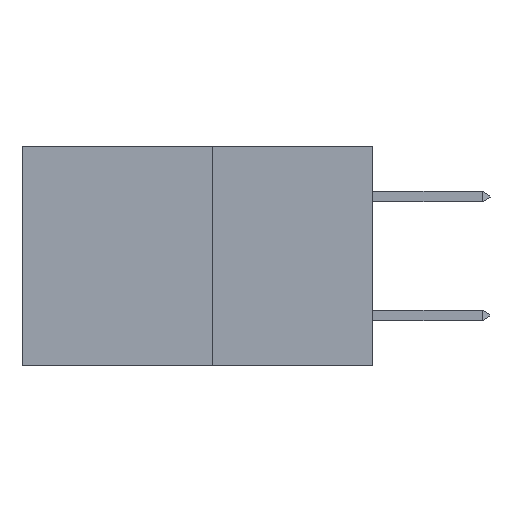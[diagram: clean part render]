
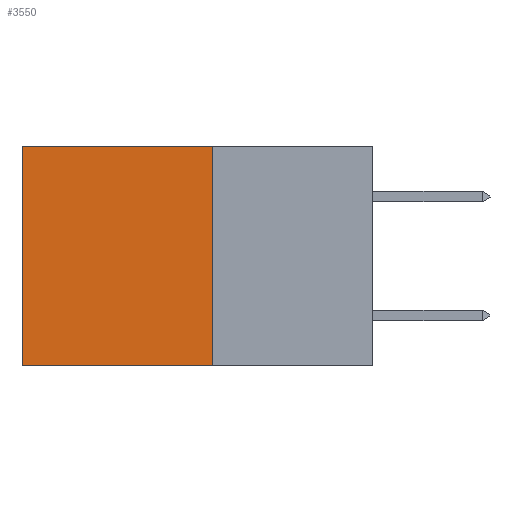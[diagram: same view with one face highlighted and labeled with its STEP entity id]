
A CAD part, left-side view. The second image highlights one B-rep face of the part: STEP entity #3550.
In plain terms, the highlighted planar face has unit normal (-1, 0, 0).
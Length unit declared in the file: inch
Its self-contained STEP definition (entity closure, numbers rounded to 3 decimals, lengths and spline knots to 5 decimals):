
#51 = CARTESIAN_POINT ( 'NONE',  ( 0.277, 0.27, -0.37 ) ) ;
#347 = LINE ( 'NONE', #5364, #7031 ) ;
#578 = EDGE_CURVE ( 'NONE', #8061, #8725, #347, .T. ) ;
#642 = EDGE_CURVE ( 'NONE', #658, #8061, #9654, .T. ) ;
#658 = VERTEX_POINT ( 'NONE', #11621 ) ;
#836 = ORIENTED_EDGE ( 'NONE', *, *, #642, .T. ) ;
#2656 = VECTOR ( 'NONE', #3033, 39.37008 ) ;
#2782 = DIRECTION ( 'NONE',  ( 0., 0., -1. ) ) ;
#3033 = DIRECTION ( 'NONE',  ( 0., 1., 0. ) ) ;
#3070 = ORIENTED_EDGE ( 'NONE', *, *, #578, .T. ) ;
#3172 = ORIENTED_EDGE ( 'NONE', *, *, #9433, .F. ) ;
#3295 = CARTESIAN_POINT ( 'NONE',  ( 0.277, 0.27, -0.37 ) ) ;
#3550 = ADVANCED_FACE ( 'NONE', ( #11007 ), #14685, .F. ) ;
#3627 = VERTEX_POINT ( 'NONE', #3295 ) ;
#4628 = EDGE_CURVE ( 'NONE', #658, #3627, #12767, .T. ) ;
#5364 = CARTESIAN_POINT ( 'NONE',  ( 0.277, 0.59, -0.37 ) ) ;
#6487 = ORIENTED_EDGE ( 'NONE', *, *, #4628, .F. ) ;
#7031 = VECTOR ( 'NONE', #2782, 39.37008 ) ;
#7602 = DIRECTION ( 'NONE',  ( 1., 0., 0. ) ) ;
#8047 = DIRECTION ( 'NONE',  ( 0., 1., 0. ) ) ;
#8061 = VERTEX_POINT ( 'NONE', #11610 ) ;
#8725 = VERTEX_POINT ( 'NONE', #16346 ) ;
#9433 = EDGE_CURVE ( 'NONE', #3627, #8725, #15487, .T. ) ;
#9654 = LINE ( 'NONE', #13429, #2656 ) ;
#11007 = FACE_OUTER_BOUND ( 'NONE', #14581, .T. ) ;
#11352 = AXIS2_PLACEMENT_3D ( 'NONE', #14327, #7602, #15580 ) ;
#11610 = CARTESIAN_POINT ( 'NONE',  ( 0.277, 0.59, 0. ) ) ;
#11621 = CARTESIAN_POINT ( 'NONE',  ( 0.277, 0.27, 0. ) ) ;
#12380 = VECTOR ( 'NONE', #14485, 39.37008 ) ;
#12767 = LINE ( 'NONE', #14784, #12380 ) ;
#13429 = CARTESIAN_POINT ( 'NONE',  ( 0.277, 0.27, 0. ) ) ;
#14327 = CARTESIAN_POINT ( 'NONE',  ( 0.277, 0.27, -0.37 ) ) ;
#14485 = DIRECTION ( 'NONE',  ( 0., 0., -1. ) ) ;
#14581 = EDGE_LOOP ( 'NONE', ( #3070, #3172, #6487, #836 ) ) ;
#14685 = PLANE ( 'NONE',  #11352 ) ;
#14784 = CARTESIAN_POINT ( 'NONE',  ( 0.277, 0.27, -0.37 ) ) ;
#15487 = LINE ( 'NONE', #51, #15891 ) ;
#15580 = DIRECTION ( 'NONE',  ( 0., 0., -1. ) ) ;
#15891 = VECTOR ( 'NONE', #8047, 39.37008 ) ;
#16346 = CARTESIAN_POINT ( 'NONE',  ( 0.277, 0.59, -0.37 ) ) ;
